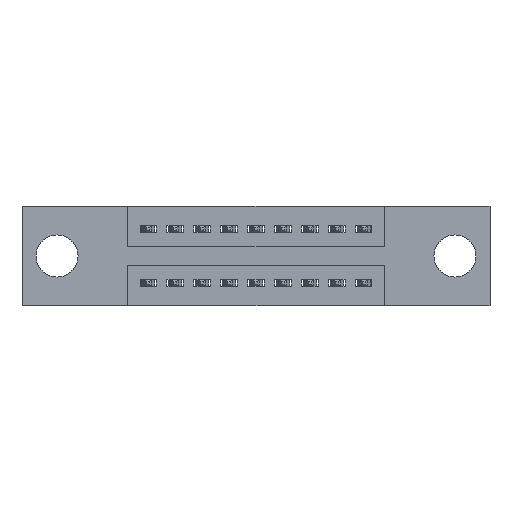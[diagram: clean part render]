
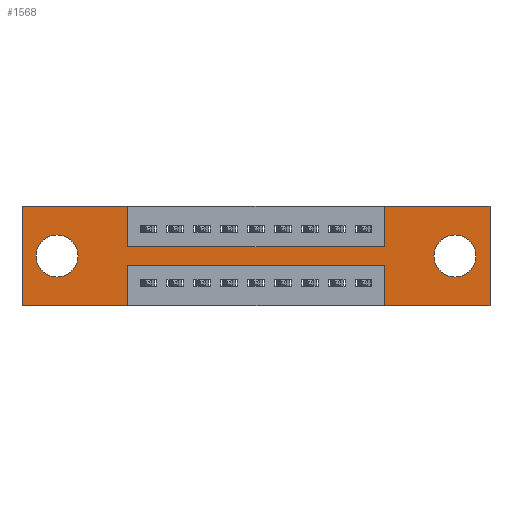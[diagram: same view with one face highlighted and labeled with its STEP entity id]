
A CAD part, front view. The second image highlights one B-rep face of the part: STEP entity #1568.
In plain terms, the highlighted planar face has unit normal (0, -1, 0).
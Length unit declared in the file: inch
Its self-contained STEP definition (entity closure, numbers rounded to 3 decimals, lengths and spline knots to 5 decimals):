
#67 = CARTESIAN_POINT ( 'NONE',  ( 1.735, 0., -0.37 ) ) ;
#79 = VERTEX_POINT ( 'NONE', #9795 ) ;
#346 = ORIENTED_EDGE ( 'NONE', *, *, #10471, .F. ) ;
#347 = DIRECTION ( 'NONE',  ( -1., 0., 0. ) ) ;
#351 = ORIENTED_EDGE ( 'NONE', *, *, #7422, .F. ) ;
#389 = CARTESIAN_POINT ( 'NONE',  ( 1.605, 0., -0.185 ) ) ;
#463 = ORIENTED_EDGE ( 'NONE', *, *, #4083, .F. ) ;
#504 = CIRCLE ( 'NONE', #10755, 0.078 ) ;
#521 = AXIS2_PLACEMENT_3D ( 'NONE', #389, #6873, #1440 ) ;
#600 = VECTOR ( 'NONE', #3277, 39.37008 ) ;
#625 = ORIENTED_EDGE ( 'NONE', *, *, #10960, .F. ) ;
#639 = ORIENTED_EDGE ( 'NONE', *, *, #3663, .T. ) ;
#687 = CARTESIAN_POINT ( 'NONE',  ( 0., 0., -0.37 ) ) ;
#751 = CARTESIAN_POINT ( 'NONE',  ( 0.13, 0., -0.185 ) ) ;
#858 = CARTESIAN_POINT ( 'NONE',  ( 0.13, 0., -0.185 ) ) ;
#1148 = VECTOR ( 'NONE', #347, 39.37008 ) ;
#1244 = DIRECTION ( 'NONE',  ( 0., -1., 0. ) ) ;
#1318 = ORIENTED_EDGE ( 'NONE', *, *, #1513, .F. ) ;
#1408 = VECTOR ( 'NONE', #3368, 39.37008 ) ;
#1440 = DIRECTION ( 'NONE',  ( 0., 0., -1. ) ) ;
#1513 = EDGE_CURVE ( 'NONE', #11494, #9334, #5222, .T. ) ;
#1568 = ADVANCED_FACE ( 'NONE', ( #2954, #9622, #5116 ), #9919, .T. ) ;
#1623 = DIRECTION ( 'NONE',  ( 0., 0., -1. ) ) ;
#1646 = CARTESIAN_POINT ( 'NONE',  ( 0.3925, 0., -0.15 ) ) ;
#1806 = DIRECTION ( 'NONE',  ( 0., 0., 1. ) ) ;
#1809 = CARTESIAN_POINT ( 'NONE',  ( 1.3425, 0., 0. ) ) ;
#1883 = VERTEX_POINT ( 'NONE', #8899 ) ;
#1917 = DIRECTION ( 'NONE',  ( 0., 0., 1. ) ) ;
#1980 = DIRECTION ( 'NONE',  ( 1., 0., 0. ) ) ;
#1984 = CARTESIAN_POINT ( 'NONE',  ( 0.3925, 0., -0.22 ) ) ;
#2013 = CARTESIAN_POINT ( 'NONE',  ( 0.3925, 0., -0.37 ) ) ;
#2103 = LINE ( 'NONE', #2311, #4575 ) ;
#2212 = CIRCLE ( 'NONE', #521, 0.078 ) ;
#2311 = CARTESIAN_POINT ( 'NONE',  ( 0., 0., 0. ) ) ;
#2316 = CARTESIAN_POINT ( 'NONE',  ( 1.735, 0., 0. ) ) ;
#2334 = CARTESIAN_POINT ( 'NONE',  ( 0., 0., -0.37 ) ) ;
#2397 = CARTESIAN_POINT ( 'NONE',  ( 0., 0., 0. ) ) ;
#2400 = CARTESIAN_POINT ( 'NONE',  ( 0., 0., -0.37 ) ) ;
#2422 = DIRECTION ( 'NONE',  ( -1., 0., 0. ) ) ;
#2495 = VECTOR ( 'NONE', #1980, 39.37008 ) ;
#2740 = VERTEX_POINT ( 'NONE', #8314 ) ;
#2798 = LINE ( 'NONE', #9811, #2495 ) ;
#2835 = VERTEX_POINT ( 'NONE', #7860 ) ;
#2932 = LINE ( 'NONE', #1809, #5091 ) ;
#2954 = FACE_BOUND ( 'NONE', #11044, .T. ) ;
#3277 = DIRECTION ( 'NONE',  ( 0., 0., -1. ) ) ;
#3280 = EDGE_CURVE ( 'NONE', #8216, #10574, #8487, .T. ) ;
#3337 = ORIENTED_EDGE ( 'NONE', *, *, #11292, .F. ) ;
#3341 = VERTEX_POINT ( 'NONE', #1646 ) ;
#3343 = DIRECTION ( 'NONE',  ( 0., 0., -1. ) ) ;
#3368 = DIRECTION ( 'NONE',  ( 0., 0., 1. ) ) ;
#3439 = CARTESIAN_POINT ( 'NONE',  ( 0., 0., 0. ) ) ;
#3663 = EDGE_CURVE ( 'NONE', #2835, #2740, #504, .T. ) ;
#3731 = LINE ( 'NONE', #5164, #1148 ) ;
#3762 = CARTESIAN_POINT ( 'NONE',  ( 0.3925, 0., 0. ) ) ;
#3874 = VECTOR ( 'NONE', #2422, 39.37008 ) ;
#4024 = CARTESIAN_POINT ( 'NONE',  ( 0., 0., -0.37 ) ) ;
#4027 = AXIS2_PLACEMENT_3D ( 'NONE', #4680, #10608, #5584 ) ;
#4030 = VECTOR ( 'NONE', #8970, 39.37008 ) ;
#4083 = EDGE_CURVE ( 'NONE', #8580, #6302, #2103, .T. ) ;
#4136 = EDGE_CURVE ( 'NONE', #10424, #6395, #3731, .T. ) ;
#4272 = ORIENTED_EDGE ( 'NONE', *, *, #5465, .T. ) ;
#4305 = CIRCLE ( 'NONE', #4027, 0.078 ) ;
#4394 = VERTEX_POINT ( 'NONE', #11236 ) ;
#4575 = VECTOR ( 'NONE', #8492, 39.37008 ) ;
#4680 = CARTESIAN_POINT ( 'NONE',  ( 1.605, 0., -0.185 ) ) ;
#4941 = DIRECTION ( 'NONE',  ( -1., 0., 0. ) ) ;
#4979 = LINE ( 'NONE', #11380, #11175 ) ;
#5090 = AXIS2_PLACEMENT_3D ( 'NONE', #687, #1244, #1623 ) ;
#5091 = VECTOR ( 'NONE', #8882, 39.37008 ) ;
#5116 = FACE_OUTER_BOUND ( 'NONE', #5831, .T. ) ;
#5150 = CARTESIAN_POINT ( 'NONE',  ( 0.3925, 0., 0. ) ) ;
#5164 = CARTESIAN_POINT ( 'NONE',  ( 0.3925, 0., -0.22 ) ) ;
#5222 = LINE ( 'NONE', #4024, #9467 ) ;
#5400 = DIRECTION ( 'NONE',  ( 0., 0., -1. ) ) ;
#5465 = EDGE_CURVE ( 'NONE', #1883, #4394, #4305, .T. ) ;
#5539 = VERTEX_POINT ( 'NONE', #5661 ) ;
#5573 = CARTESIAN_POINT ( 'NONE',  ( 0., 0., 0. ) ) ;
#5584 = DIRECTION ( 'NONE',  ( 0., 0., -1. ) ) ;
#5661 = CARTESIAN_POINT ( 'NONE',  ( 1.3425, 0., -0.15 ) ) ;
#5672 = EDGE_LOOP ( 'NONE', ( #6842, #639 ) ) ;
#5718 = ORIENTED_EDGE ( 'NONE', *, *, #10599, .F. ) ;
#5829 = ORIENTED_EDGE ( 'NONE', *, *, #6127, .F. ) ;
#5831 = EDGE_LOOP ( 'NONE', ( #5829, #8868, #10428, #9418, #9676, #346, #3337, #5718, #351, #463, #625, #1318 ) ) ;
#5937 = LINE ( 'NONE', #5150, #600 ) ;
#6076 = VERTEX_POINT ( 'NONE', #6996 ) ;
#6093 = VECTOR ( 'NONE', #5400, 39.37008 ) ;
#6127 = EDGE_CURVE ( 'NONE', #6395, #11494, #8306, .T. ) ;
#6270 = EDGE_CURVE ( 'NONE', #10574, #10424, #4979, .T. ) ;
#6302 = VERTEX_POINT ( 'NONE', #3762 ) ;
#6313 = LINE ( 'NONE', #2397, #1408 ) ;
#6385 = LINE ( 'NONE', #5573, #4030 ) ;
#6395 = VERTEX_POINT ( 'NONE', #1984 ) ;
#6784 = EDGE_CURVE ( 'NONE', #4394, #1883, #2212, .T. ) ;
#6842 = ORIENTED_EDGE ( 'NONE', *, *, #8801, .T. ) ;
#6873 = DIRECTION ( 'NONE',  ( 0., 1., 0. ) ) ;
#6996 = CARTESIAN_POINT ( 'NONE',  ( 1.3425, 0., 0. ) ) ;
#7145 = DIRECTION ( 'NONE',  ( 0., 1., 0. ) ) ;
#7201 = DIRECTION ( 'NONE',  ( 0., 0., 1. ) ) ;
#7222 = AXIS2_PLACEMENT_3D ( 'NONE', #751, #7145, #1806 ) ;
#7243 = DIRECTION ( 'NONE',  ( 0., 1., 0. ) ) ;
#7422 = EDGE_CURVE ( 'NONE', #6302, #3341, #5937, .T. ) ;
#7860 = CARTESIAN_POINT ( 'NONE',  ( 0.13, 0., -0.263 ) ) ;
#8216 = VERTEX_POINT ( 'NONE', #67 ) ;
#8306 = LINE ( 'NONE', #11247, #6093 ) ;
#8314 = CARTESIAN_POINT ( 'NONE',  ( 0.13, 0., -0.107 ) ) ;
#8487 = LINE ( 'NONE', #2400, #3874 ) ;
#8492 = DIRECTION ( 'NONE',  ( 1., 0., 0. ) ) ;
#8580 = VERTEX_POINT ( 'NONE', #3439 ) ;
#8777 = VECTOR ( 'NONE', #3343, 39.37008 ) ;
#8801 = EDGE_CURVE ( 'NONE', #2740, #2835, #9717, .T. ) ;
#8848 = ORIENTED_EDGE ( 'NONE', *, *, #6784, .T. ) ;
#8868 = ORIENTED_EDGE ( 'NONE', *, *, #4136, .F. ) ;
#8882 = DIRECTION ( 'NONE',  ( 0., 0., 1. ) ) ;
#8899 = CARTESIAN_POINT ( 'NONE',  ( 1.605, 0., -0.107 ) ) ;
#8970 = DIRECTION ( 'NONE',  ( 1., 0., 0. ) ) ;
#9334 = VERTEX_POINT ( 'NONE', #2334 ) ;
#9418 = ORIENTED_EDGE ( 'NONE', *, *, #3280, .F. ) ;
#9467 = VECTOR ( 'NONE', #4941, 39.37008 ) ;
#9622 = FACE_BOUND ( 'NONE', #5672, .T. ) ;
#9676 = ORIENTED_EDGE ( 'NONE', *, *, #10198, .F. ) ;
#9717 = CIRCLE ( 'NONE', #7222, 0.078 ) ;
#9795 = CARTESIAN_POINT ( 'NONE',  ( 1.735, 0., 0. ) ) ;
#9811 = CARTESIAN_POINT ( 'NONE',  ( 0.3925, 0., -0.15 ) ) ;
#9919 = PLANE ( 'NONE',  #5090 ) ;
#10198 = EDGE_CURVE ( 'NONE', #79, #8216, #11219, .T. ) ;
#10424 = VERTEX_POINT ( 'NONE', #11379 ) ;
#10428 = ORIENTED_EDGE ( 'NONE', *, *, #6270, .F. ) ;
#10471 = EDGE_CURVE ( 'NONE', #6076, #79, #6385, .T. ) ;
#10574 = VERTEX_POINT ( 'NONE', #10703 ) ;
#10599 = EDGE_CURVE ( 'NONE', #3341, #5539, #2798, .T. ) ;
#10608 = DIRECTION ( 'NONE',  ( 0., 1., 0. ) ) ;
#10703 = CARTESIAN_POINT ( 'NONE',  ( 1.3425, 0., -0.37 ) ) ;
#10755 = AXIS2_PLACEMENT_3D ( 'NONE', #858, #7243, #1917 ) ;
#10960 = EDGE_CURVE ( 'NONE', #9334, #8580, #6313, .T. ) ;
#11044 = EDGE_LOOP ( 'NONE', ( #4272, #8848 ) ) ;
#11175 = VECTOR ( 'NONE', #7201, 39.37008 ) ;
#11219 = LINE ( 'NONE', #2316, #8777 ) ;
#11236 = CARTESIAN_POINT ( 'NONE',  ( 1.605, 0., -0.263 ) ) ;
#11247 = CARTESIAN_POINT ( 'NONE',  ( 0.3925, 0., -0.37 ) ) ;
#11292 = EDGE_CURVE ( 'NONE', #5539, #6076, #2932, .T. ) ;
#11379 = CARTESIAN_POINT ( 'NONE',  ( 1.3425, 0., -0.22 ) ) ;
#11380 = CARTESIAN_POINT ( 'NONE',  ( 1.3425, 0., -0.37 ) ) ;
#11494 = VERTEX_POINT ( 'NONE', #2013 ) ;
